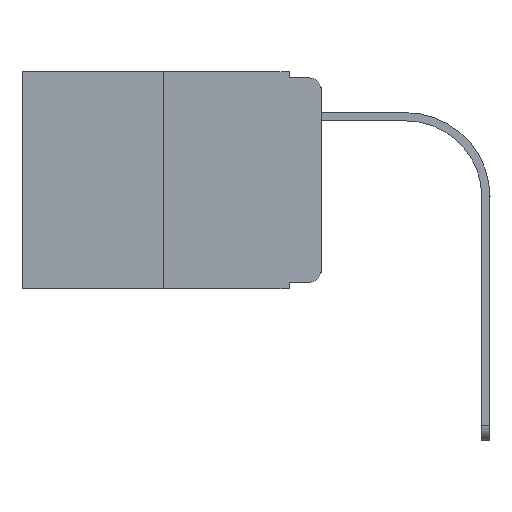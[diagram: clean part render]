
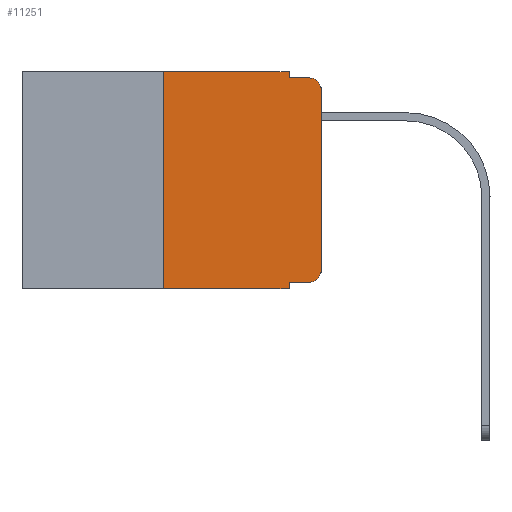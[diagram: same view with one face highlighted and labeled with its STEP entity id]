
A CAD part, left-side view. The second image highlights one B-rep face of the part: STEP entity #11251.
In plain terms, the highlighted planar face has unit normal (-1, 0, 0).
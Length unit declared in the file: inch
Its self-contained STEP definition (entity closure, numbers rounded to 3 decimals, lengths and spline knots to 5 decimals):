
#348 = DIRECTION ( 'NONE',  ( 0., 0., 1. ) ) ;
#929 = VECTOR ( 'NONE', #11890, 39.37008 ) ;
#1041 = EDGE_CURVE ( 'NONE', #11499, #10222, #6816, .T. ) ;
#1275 = CARTESIAN_POINT ( 'NONE',  ( 0., 0.051, 0. ) ) ;
#1334 = LINE ( 'NONE', #3460, #929 ) ;
#1402 = EDGE_CURVE ( 'NONE', #13602, #2435, #3694, .T. ) ;
#1539 = DIRECTION ( 'NONE',  ( 1., 0., 0. ) ) ;
#1604 = EDGE_CURVE ( 'NONE', #4135, #1902, #1959, .T. ) ;
#1737 = ORIENTED_EDGE ( 'NONE', *, *, #4156, .F. ) ;
#1902 = VERTEX_POINT ( 'NONE', #11901 ) ;
#1959 = LINE ( 'NONE', #10979, #10395 ) ;
#2100 = ORIENTED_EDGE ( 'NONE', *, *, #1041, .T. ) ;
#2435 = VERTEX_POINT ( 'NONE', #8068 ) ;
#2464 = ORIENTED_EDGE ( 'NONE', *, *, #13359, .F. ) ;
#2617 = LINE ( 'NONE', #4680, #8977 ) ;
#2749 = VERTEX_POINT ( 'NONE', #14162 ) ;
#2880 = VECTOR ( 'NONE', #11238, 39.37008 ) ;
#2970 = CARTESIAN_POINT ( 'NONE',  ( 0., 0.473, 0. ) ) ;
#3065 = CARTESIAN_POINT ( 'NONE',  ( 0., 0.051, -0.01 ) ) ;
#3127 = DIRECTION ( 'NONE',  ( 0., -1., 0. ) ) ;
#3186 = DIRECTION ( 'NONE',  ( 0., -1., 0. ) ) ;
#3459 = CARTESIAN_POINT ( 'NONE',  ( 0., 0.051, -0.333 ) ) ;
#3460 = CARTESIAN_POINT ( 'NONE',  ( 0., 0.051, 0. ) ) ;
#3574 = VERTEX_POINT ( 'NONE', #3065 ) ;
#3600 = CARTESIAN_POINT ( 'NONE',  ( 0., 0.473, 0. ) ) ;
#3607 = CARTESIAN_POINT ( 'NONE',  ( 0., 0.02, -0.313 ) ) ;
#3694 = LINE ( 'NONE', #13699, #3938 ) ;
#3893 = DIRECTION ( 'NONE',  ( 0., 0., -1. ) ) ;
#3938 = VECTOR ( 'NONE', #348, 39.37008 ) ;
#4099 = EDGE_CURVE ( 'NONE', #1902, #11086, #13277, .T. ) ;
#4135 = VERTEX_POINT ( 'NONE', #3459 ) ;
#4150 = ORIENTED_EDGE ( 'NONE', *, *, #14192, .F. ) ;
#4156 = EDGE_CURVE ( 'NONE', #4135, #4660, #13595, .T. ) ;
#4244 = EDGE_CURVE ( 'NONE', #11086, #11499, #6694, .T. ) ;
#4289 = EDGE_LOOP ( 'NONE', ( #13141, #2100, #2464, #4150, #12592, #11486, #8420, #1737, #7399, #6517 ) ) ;
#4528 = AXIS2_PLACEMENT_3D ( 'NONE', #3607, #13743, #5679 ) ;
#4562 = CARTESIAN_POINT ( 'NONE',  ( 0., 0., -0.03 ) ) ;
#4660 = VERTEX_POINT ( 'NONE', #5577 ) ;
#4680 = CARTESIAN_POINT ( 'NONE',  ( 0., 0.051, -0.01 ) ) ;
#4807 = VECTOR ( 'NONE', #7490, 39.37008 ) ;
#4893 = DIRECTION ( 'NONE',  ( 0., -1., 0. ) ) ;
#5222 = AXIS2_PLACEMENT_3D ( 'NONE', #3600, #1539, #3893 ) ;
#5577 = CARTESIAN_POINT ( 'NONE',  ( 0., 0.051, -0.343 ) ) ;
#5679 = DIRECTION ( 'NONE',  ( 0., 0., -1. ) ) ;
#5683 = CARTESIAN_POINT ( 'NONE',  ( 0., 0.473, -0.343 ) ) ;
#5752 = DIRECTION ( 'NONE',  ( 0., 0., -1. ) ) ;
#6022 = FACE_OUTER_BOUND ( 'NONE', #4289, .T. ) ;
#6517 = ORIENTED_EDGE ( 'NONE', *, *, #4099, .T. ) ;
#6694 = LINE ( 'NONE', #9007, #2880 ) ;
#6816 = CIRCLE ( 'NONE', #11594, 0.02 ) ;
#6890 = VECTOR ( 'NONE', #5752, 39.37008 ) ;
#7005 = PLANE ( 'NONE',  #5222 ) ;
#7399 = ORIENTED_EDGE ( 'NONE', *, *, #1604, .T. ) ;
#7490 = DIRECTION ( 'NONE',  ( 0., -1., 0. ) ) ;
#8068 = CARTESIAN_POINT ( 'NONE',  ( 0., 0.25, 0. ) ) ;
#8420 = ORIENTED_EDGE ( 'NONE', *, *, #14061, .T. ) ;
#8977 = VECTOR ( 'NONE', #4893, 39.37008 ) ;
#9007 = CARTESIAN_POINT ( 'NONE',  ( 0., 0., 0. ) ) ;
#9557 = CARTESIAN_POINT ( 'NONE',  ( 0., 0.25, -0.343 ) ) ;
#10222 = VERTEX_POINT ( 'NONE', #13267 ) ;
#10259 = DIRECTION ( 'NONE',  ( 0., 0., -1. ) ) ;
#10395 = VECTOR ( 'NONE', #3127, 39.37008 ) ;
#10979 = CARTESIAN_POINT ( 'NONE',  ( 0., 0.051, -0.333 ) ) ;
#11086 = VERTEX_POINT ( 'NONE', #13656 ) ;
#11238 = DIRECTION ( 'NONE',  ( 0., 0., 1. ) ) ;
#11251 = ADVANCED_FACE ( 'NONE', ( #6022 ), #7005, .F. ) ;
#11486 = ORIENTED_EDGE ( 'NONE', *, *, #1402, .F. ) ;
#11499 = VERTEX_POINT ( 'NONE', #4562 ) ;
#11587 = CARTESIAN_POINT ( 'NONE',  ( 0., 0.02, -0.03 ) ) ;
#11594 = AXIS2_PLACEMENT_3D ( 'NONE', #11587, #13571, #10259 ) ;
#11870 = LINE ( 'NONE', #2970, #4807 ) ;
#11890 = DIRECTION ( 'NONE',  ( 0., 0., -1. ) ) ;
#11901 = CARTESIAN_POINT ( 'NONE',  ( 0., 0.02, -0.333 ) ) ;
#12129 = VECTOR ( 'NONE', #3186, 39.37008 ) ;
#12429 = LINE ( 'NONE', #5683, #12129 ) ;
#12592 = ORIENTED_EDGE ( 'NONE', *, *, #13488, .F. ) ;
#13141 = ORIENTED_EDGE ( 'NONE', *, *, #4244, .T. ) ;
#13267 = CARTESIAN_POINT ( 'NONE',  ( 0., 0.02, -0.01 ) ) ;
#13277 = CIRCLE ( 'NONE', #4528, 0.02 ) ;
#13359 = EDGE_CURVE ( 'NONE', #3574, #10222, #2617, .T. ) ;
#13488 = EDGE_CURVE ( 'NONE', #2435, #2749, #11870, .T. ) ;
#13571 = DIRECTION ( 'NONE',  ( -1., 0., 0. ) ) ;
#13595 = LINE ( 'NONE', #1275, #6890 ) ;
#13602 = VERTEX_POINT ( 'NONE', #9557 ) ;
#13656 = CARTESIAN_POINT ( 'NONE',  ( 0., 0., -0.313 ) ) ;
#13699 = CARTESIAN_POINT ( 'NONE',  ( 0., 0.25, 0. ) ) ;
#13743 = DIRECTION ( 'NONE',  ( -1., 0., 0. ) ) ;
#14061 = EDGE_CURVE ( 'NONE', #13602, #4660, #12429, .T. ) ;
#14162 = CARTESIAN_POINT ( 'NONE',  ( 0., 0.051, 0. ) ) ;
#14192 = EDGE_CURVE ( 'NONE', #2749, #3574, #1334, .T. ) ;
